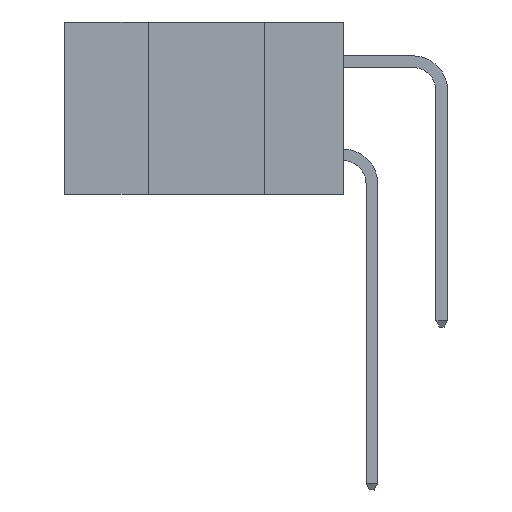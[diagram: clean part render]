
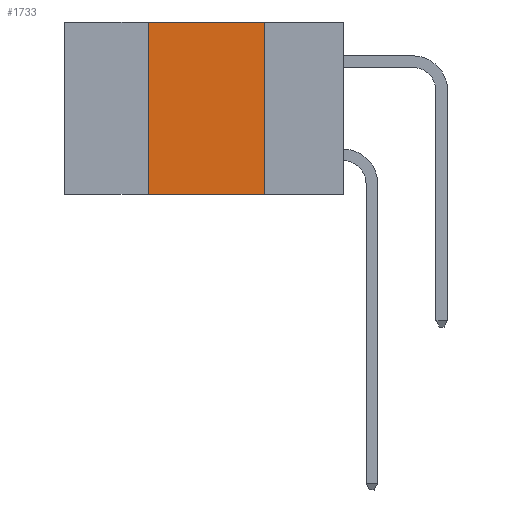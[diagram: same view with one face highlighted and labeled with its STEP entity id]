
A CAD part, left-side view. The second image highlights one B-rep face of the part: STEP entity #1733.
In plain terms, the highlighted planar face has unit normal (-1, 0, 0).
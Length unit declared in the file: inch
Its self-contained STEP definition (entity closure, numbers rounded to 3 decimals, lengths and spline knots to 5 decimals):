
#271 = DIRECTION ( 'NONE',  ( 0., -1., 0. ) ) ;
#1011 = DIRECTION ( 'NONE',  ( 1., 0., 0. ) ) ;
#1542 = ORIENTED_EDGE ( 'NONE', *, *, #9251, .T. ) ;
#1733 = ADVANCED_FACE ( 'NONE', ( #7598 ), #8302, .F. ) ;
#2482 = VERTEX_POINT ( 'NONE', #3112 ) ;
#2810 = CARTESIAN_POINT ( 'NONE',  ( 0., 0.6, -0.37 ) ) ;
#2818 = VECTOR ( 'NONE', #271, 39.37008 ) ;
#3007 = VERTEX_POINT ( 'NONE', #6962 ) ;
#3112 = CARTESIAN_POINT ( 'NONE',  ( 0., 0.42, -0.37 ) ) ;
#3439 = EDGE_CURVE ( 'NONE', #13020, #5726, #6390, .T. ) ;
#3501 = DIRECTION ( 'NONE',  ( 0., 0., 1. ) ) ;
#4687 = ORIENTED_EDGE ( 'NONE', *, *, #3439, .F. ) ;
#5726 = VERTEX_POINT ( 'NONE', #6837 ) ;
#6211 = CARTESIAN_POINT ( 'NONE',  ( 0., 0.42, 0. ) ) ;
#6390 = LINE ( 'NONE', #6806, #8477 ) ;
#6753 = AXIS2_PLACEMENT_3D ( 'NONE', #10717, #1011, #9506 ) ;
#6806 = CARTESIAN_POINT ( 'NONE',  ( 0., 0.6, 0. ) ) ;
#6814 = EDGE_LOOP ( 'NONE', ( #9604, #4687, #13641, #1542 ) ) ;
#6837 = CARTESIAN_POINT ( 'NONE',  ( 0., 0.17, 0. ) ) ;
#6962 = CARTESIAN_POINT ( 'NONE',  ( 0., 0.17, -0.37 ) ) ;
#7013 = LINE ( 'NONE', #7159, #12933 ) ;
#7159 = CARTESIAN_POINT ( 'NONE',  ( 0., 0.42, 0. ) ) ;
#7598 = FACE_OUTER_BOUND ( 'NONE', #6814, .T. ) ;
#7903 = DIRECTION ( 'NONE',  ( 0., -1., 0. ) ) ;
#8302 = PLANE ( 'NONE',  #6753 ) ;
#8477 = VECTOR ( 'NONE', #7903, 39.37008 ) ;
#9251 = EDGE_CURVE ( 'NONE', #2482, #3007, #14424, .T. ) ;
#9506 = DIRECTION ( 'NONE',  ( 0., 0., -1. ) ) ;
#9571 = EDGE_CURVE ( 'NONE', #2482, #13020, #7013, .T. ) ;
#9604 = ORIENTED_EDGE ( 'NONE', *, *, #13702, .F. ) ;
#9896 = DIRECTION ( 'NONE',  ( 0., 0., -1. ) ) ;
#10687 = LINE ( 'NONE', #15356, #13176 ) ;
#10717 = CARTESIAN_POINT ( 'NONE',  ( 0., 0.6, 0. ) ) ;
#12933 = VECTOR ( 'NONE', #3501, 39.37008 ) ;
#13020 = VERTEX_POINT ( 'NONE', #6211 ) ;
#13176 = VECTOR ( 'NONE', #9896, 39.37008 ) ;
#13641 = ORIENTED_EDGE ( 'NONE', *, *, #9571, .F. ) ;
#13702 = EDGE_CURVE ( 'NONE', #5726, #3007, #10687, .T. ) ;
#14424 = LINE ( 'NONE', #2810, #2818 ) ;
#15356 = CARTESIAN_POINT ( 'NONE',  ( 0., 0.17, 0. ) ) ;
